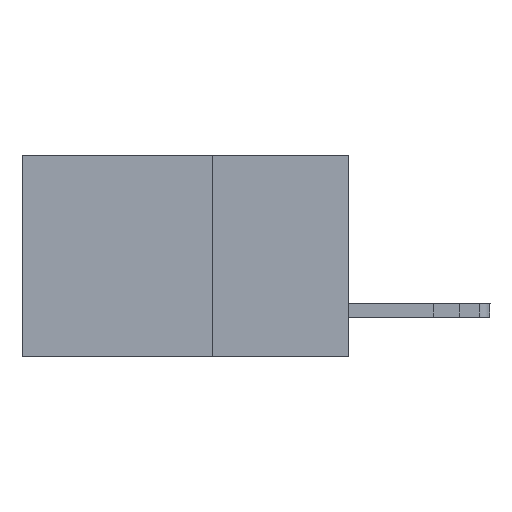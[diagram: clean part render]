
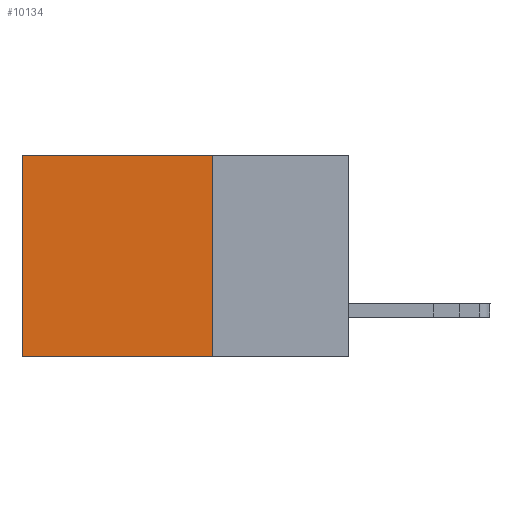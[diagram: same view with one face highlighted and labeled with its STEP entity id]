
A CAD part, left-side view. The second image highlights one B-rep face of the part: STEP entity #10134.
In plain terms, the highlighted planar face has unit normal (-1, 0, 0).
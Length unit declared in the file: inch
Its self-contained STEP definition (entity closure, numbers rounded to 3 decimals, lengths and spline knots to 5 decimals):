
#710 = DIRECTION ( 'NONE',  ( 0., 0., -1. ) ) ;
#1028 = CARTESIAN_POINT ( 'NONE',  ( 0.2615, 0.25, -0.37 ) ) ;
#1962 = VECTOR ( 'NONE', #14728, 39.37008 ) ;
#2434 = LINE ( 'NONE', #15402, #1962 ) ;
#3862 = EDGE_CURVE ( 'NONE', #15739, #15835, #2434, .T. ) ;
#3916 = DIRECTION ( 'NONE',  ( 0., 1., 0. ) ) ;
#3938 = DIRECTION ( 'NONE',  ( 0., 1., 0. ) ) ;
#4277 = CARTESIAN_POINT ( 'NONE',  ( 0.2615, 0.25, -0.37 ) ) ;
#4391 = EDGE_CURVE ( 'NONE', #14600, #14052, #16109, .T. ) ;
#4789 = CARTESIAN_POINT ( 'NONE',  ( 0.2615, 0.25, -0.37 ) ) ;
#5441 = VECTOR ( 'NONE', #3938, 39.37008 ) ;
#5621 = CARTESIAN_POINT ( 'NONE',  ( 0.2615, 0.6, 0. ) ) ;
#5809 = CARTESIAN_POINT ( 'NONE',  ( 0.2615, 0.6, -0.37 ) ) ;
#6175 = DIRECTION ( 'NONE',  ( 1., 0., 0. ) ) ;
#6638 = LINE ( 'NONE', #12333, #9935 ) ;
#6865 = CARTESIAN_POINT ( 'NONE',  ( 0.2615, 0.25, 0. ) ) ;
#8105 = ORIENTED_EDGE ( 'NONE', *, *, #4391, .F. ) ;
#8722 = ORIENTED_EDGE ( 'NONE', *, *, #12732, .T. ) ;
#9730 = EDGE_CURVE ( 'NONE', #14052, #15835, #6638, .T. ) ;
#9935 = VECTOR ( 'NONE', #3916, 39.37008 ) ;
#10134 = ADVANCED_FACE ( 'NONE', ( #13918 ), #13088, .F. ) ;
#12146 = VECTOR ( 'NONE', #710, 39.37008 ) ;
#12333 = CARTESIAN_POINT ( 'NONE',  ( 0.2615, 0.25, -0.37 ) ) ;
#12732 = EDGE_CURVE ( 'NONE', #14600, #15739, #16348, .T. ) ;
#13088 = PLANE ( 'NONE',  #14067 ) ;
#13918 = FACE_OUTER_BOUND ( 'NONE', #15963, .T. ) ;
#14052 = VERTEX_POINT ( 'NONE', #4277 ) ;
#14067 = AXIS2_PLACEMENT_3D ( 'NONE', #4789, #6175, #15760 ) ;
#14600 = VERTEX_POINT ( 'NONE', #6865 ) ;
#14728 = DIRECTION ( 'NONE',  ( 0., 0., -1. ) ) ;
#14768 = ORIENTED_EDGE ( 'NONE', *, *, #9730, .F. ) ;
#14921 = ORIENTED_EDGE ( 'NONE', *, *, #3862, .T. ) ;
#15402 = CARTESIAN_POINT ( 'NONE',  ( 0.2615, 0.6, -0.37 ) ) ;
#15739 = VERTEX_POINT ( 'NONE', #5621 ) ;
#15760 = DIRECTION ( 'NONE',  ( 0., 0., -1. ) ) ;
#15835 = VERTEX_POINT ( 'NONE', #5809 ) ;
#15963 = EDGE_LOOP ( 'NONE', ( #14921, #14768, #8105, #8722 ) ) ;
#16109 = LINE ( 'NONE', #1028, #12146 ) ;
#16300 = CARTESIAN_POINT ( 'NONE',  ( 0.2615, 0.25, 0. ) ) ;
#16348 = LINE ( 'NONE', #16300, #5441 ) ;
